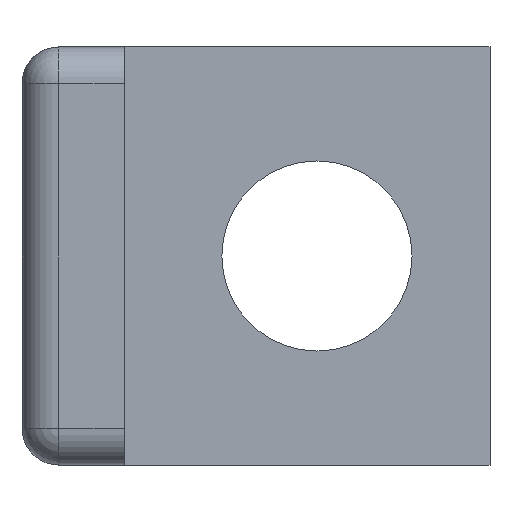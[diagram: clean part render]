
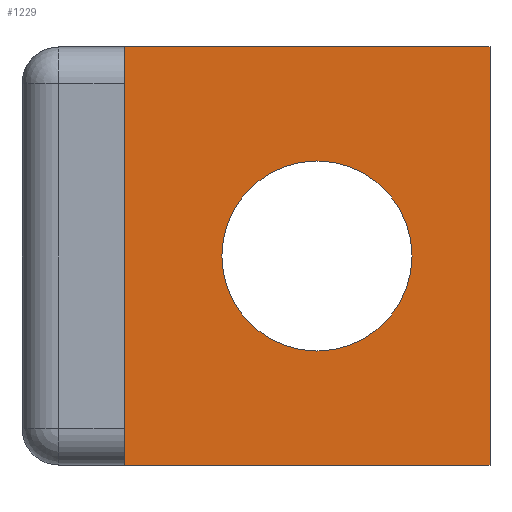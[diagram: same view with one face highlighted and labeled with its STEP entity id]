
A CAD part, front view. The second image highlights one B-rep face of the part: STEP entity #1229.
In plain terms, the highlighted planar face has unit normal (0, -1, 0).
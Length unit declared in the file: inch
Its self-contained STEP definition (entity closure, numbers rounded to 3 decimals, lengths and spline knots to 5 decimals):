
#11 = VERTEX_POINT ( 'NONE', #1126 ) ;
#15 = DIRECTION ( 'NONE',  ( 0., -1., 0. ) ) ;
#29 = AXIS2_PLACEMENT_3D ( 'NONE', #1363, #1370, #1241 ) ;
#72 = LINE ( 'NONE', #1451, #325 ) ;
#80 = DIRECTION ( 'NONE',  ( 0., 0., 1. ) ) ;
#112 = CARTESIAN_POINT ( 'NONE',  ( 0.384, 0.245, 0. ) ) ;
#141 = ORIENTED_EDGE ( 'NONE', *, *, #210, .F. ) ;
#176 = AXIS2_PLACEMENT_3D ( 'NONE', #1266, #15, #921 ) ;
#202 = VECTOR ( 'NONE', #587, 39.37008 ) ;
#210 = EDGE_CURVE ( 'NONE', #931, #1110, #1333, .T. ) ;
#221 = VERTEX_POINT ( 'NONE', #112 ) ;
#250 = VECTOR ( 'NONE', #572, 39.37008 ) ;
#283 = FACE_OUTER_BOUND ( 'NONE', #500, .T. ) ;
#305 = AXIS2_PLACEMENT_3D ( 'NONE', #855, #655, #648 ) ;
#325 = VECTOR ( 'NONE', #80, 39.37008 ) ;
#420 = DIRECTION ( 'NONE',  ( 0., 0., 1. ) ) ;
#474 = VERTEX_POINT ( 'NONE', #1323 ) ;
#479 = EDGE_CURVE ( 'NONE', #11, #221, #72, .T. ) ;
#500 = EDGE_LOOP ( 'NONE', ( #574, #828, #1032, #1098 ) ) ;
#538 = EDGE_CURVE ( 'NONE', #1110, #931, #638, .T. ) ;
#572 = DIRECTION ( 'NONE',  ( 1., 0., 0. ) ) ;
#574 = ORIENTED_EDGE ( 'NONE', *, *, #755, .F. ) ;
#581 = CARTESIAN_POINT ( 'NONE',  ( 0.384, 0.245, 0. ) ) ;
#587 = DIRECTION ( 'NONE',  ( 1., 0., 0. ) ) ;
#638 = CIRCLE ( 'NONE', #176, 0.078 ) ;
#648 = DIRECTION ( 'NONE',  ( 1., 0., 0. ) ) ;
#655 = DIRECTION ( 'NONE',  ( 0., -1., 0. ) ) ;
#672 = ORIENTED_EDGE ( 'NONE', *, *, #538, .F. ) ;
#685 = CARTESIAN_POINT ( 'NONE',  ( 0.242, 0.245, -0.2495 ) ) ;
#696 = EDGE_LOOP ( 'NONE', ( #141, #672 ) ) ;
#739 = LINE ( 'NONE', #1489, #250 ) ;
#755 = EDGE_CURVE ( 'NONE', #474, #221, #923, .T. ) ;
#828 = ORIENTED_EDGE ( 'NONE', *, *, #1419, .F. ) ;
#855 = CARTESIAN_POINT ( 'NONE',  ( 0.384, 0.245, -0.343 ) ) ;
#921 = DIRECTION ( 'NONE',  ( 1., 0., 0. ) ) ;
#923 = LINE ( 'NONE', #581, #202 ) ;
#931 = VERTEX_POINT ( 'NONE', #1107 ) ;
#971 = PLANE ( 'NONE',  #305 ) ;
#1011 = VERTEX_POINT ( 'NONE', #1471 ) ;
#1032 = ORIENTED_EDGE ( 'NONE', *, *, #1153, .T. ) ;
#1067 = CARTESIAN_POINT ( 'NONE',  ( 0.084, 0.245, -0.343 ) ) ;
#1098 = ORIENTED_EDGE ( 'NONE', *, *, #479, .T. ) ;
#1107 = CARTESIAN_POINT ( 'NONE',  ( 0.242, 0.245, -0.0935 ) ) ;
#1110 = VERTEX_POINT ( 'NONE', #685 ) ;
#1126 = CARTESIAN_POINT ( 'NONE',  ( 0.384, 0.245, -0.343 ) ) ;
#1143 = VECTOR ( 'NONE', #420, 39.37008 ) ;
#1153 = EDGE_CURVE ( 'NONE', #1011, #11, #739, .T. ) ;
#1177 = LINE ( 'NONE', #1067, #1143 ) ;
#1229 = ADVANCED_FACE ( 'NONE', ( #1448, #283 ), #971, .T. ) ;
#1241 = DIRECTION ( 'NONE',  ( 1., 0., 0. ) ) ;
#1266 = CARTESIAN_POINT ( 'NONE',  ( 0.242, 0.245, -0.1715 ) ) ;
#1323 = CARTESIAN_POINT ( 'NONE',  ( 0.084, 0.245, 0. ) ) ;
#1333 = CIRCLE ( 'NONE', #29, 0.078 ) ;
#1363 = CARTESIAN_POINT ( 'NONE',  ( 0.242, 0.245, -0.1715 ) ) ;
#1370 = DIRECTION ( 'NONE',  ( 0., -1., 0. ) ) ;
#1419 = EDGE_CURVE ( 'NONE', #1011, #474, #1177, .T. ) ;
#1448 = FACE_BOUND ( 'NONE', #696, .T. ) ;
#1451 = CARTESIAN_POINT ( 'NONE',  ( 0.384, 0.245, -0.343 ) ) ;
#1471 = CARTESIAN_POINT ( 'NONE',  ( 0.084, 0.245, -0.343 ) ) ;
#1489 = CARTESIAN_POINT ( 'NONE',  ( 0.384, 0.245, -0.343 ) ) ;
